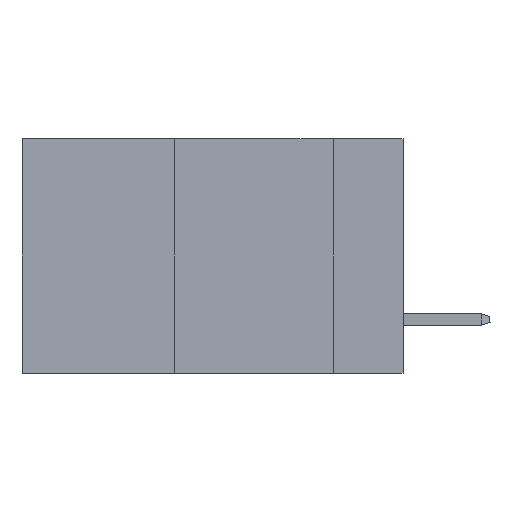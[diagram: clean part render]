
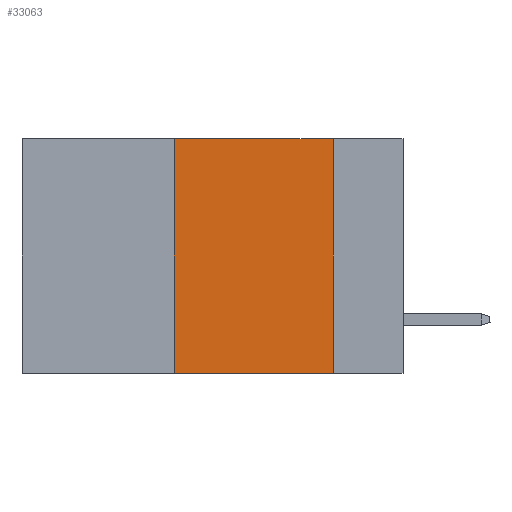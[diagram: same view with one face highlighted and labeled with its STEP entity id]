
A CAD part, left-side view. The second image highlights one B-rep face of the part: STEP entity #33063.
In plain terms, the highlighted planar face has unit normal (-1, 0, 0).
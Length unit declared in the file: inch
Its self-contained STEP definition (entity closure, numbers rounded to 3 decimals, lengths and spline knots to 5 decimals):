
#2587 = AXIS2_PLACEMENT_3D ( 'NONE', #7701, #29586, #21492 ) ;
#3029 = CARTESIAN_POINT ( 'NONE',  ( 0., 0.36, -0.37 ) ) ;
#4555 = ORIENTED_EDGE ( 'NONE', *, *, #9800, .F. ) ;
#4723 = VECTOR ( 'NONE', #30569, 39.37008 ) ;
#5368 = DIRECTION ( 'NONE',  ( 0., -1., 0. ) ) ;
#7594 = VERTEX_POINT ( 'NONE', #3029 ) ;
#7701 = CARTESIAN_POINT ( 'NONE',  ( 0., 0.6, 0. ) ) ;
#7970 = DIRECTION ( 'NONE',  ( 0., 0., 1. ) ) ;
#8715 = CARTESIAN_POINT ( 'NONE',  ( 0., 0.36, 0. ) ) ;
#9434 = VECTOR ( 'NONE', #33396, 39.37008 ) ;
#9800 = EDGE_CURVE ( 'NONE', #7594, #21122, #24262, .T. ) ;
#10902 = CARTESIAN_POINT ( 'NONE',  ( 0., 0.11, -0.37 ) ) ;
#12547 = EDGE_CURVE ( 'NONE', #25622, #34567, #19617, .T. ) ;
#13004 = CARTESIAN_POINT ( 'NONE',  ( 0., 0.36, 0. ) ) ;
#13095 = FACE_OUTER_BOUND ( 'NONE', #35415, .T. ) ;
#13695 = ORIENTED_EDGE ( 'NONE', *, *, #12547, .F. ) ;
#14243 = CARTESIAN_POINT ( 'NONE',  ( 0., 0.11, 0. ) ) ;
#15409 = EDGE_CURVE ( 'NONE', #21122, #25622, #27994, .T. ) ;
#17820 = VECTOR ( 'NONE', #7970, 39.37008 ) ;
#19617 = LINE ( 'NONE', #14243, #4723 ) ;
#19908 = CARTESIAN_POINT ( 'NONE',  ( 0., 0.6, 0. ) ) ;
#20350 = ORIENTED_EDGE ( 'NONE', *, *, #15409, .F. ) ;
#21122 = VERTEX_POINT ( 'NONE', #8715 ) ;
#21323 = PLANE ( 'NONE',  #2587 ) ;
#21492 = DIRECTION ( 'NONE',  ( 0., 0., -1. ) ) ;
#24262 = LINE ( 'NONE', #13004, #17820 ) ;
#25587 = ORIENTED_EDGE ( 'NONE', *, *, #33026, .T. ) ;
#25622 = VERTEX_POINT ( 'NONE', #27530 ) ;
#27530 = CARTESIAN_POINT ( 'NONE',  ( 0., 0.11, 0. ) ) ;
#27994 = LINE ( 'NONE', #19908, #9434 ) ;
#29586 = DIRECTION ( 'NONE',  ( 1., 0., 0. ) ) ;
#29944 = CARTESIAN_POINT ( 'NONE',  ( 0., 0.6, -0.37 ) ) ;
#30569 = DIRECTION ( 'NONE',  ( 0., 0., -1. ) ) ;
#31232 = VECTOR ( 'NONE', #5368, 39.37008 ) ;
#33026 = EDGE_CURVE ( 'NONE', #7594, #34567, #35164, .T. ) ;
#33063 = ADVANCED_FACE ( 'NONE', ( #13095 ), #21323, .F. ) ;
#33396 = DIRECTION ( 'NONE',  ( 0., -1., 0. ) ) ;
#34567 = VERTEX_POINT ( 'NONE', #10902 ) ;
#35164 = LINE ( 'NONE', #29944, #31232 ) ;
#35415 = EDGE_LOOP ( 'NONE', ( #13695, #20350, #4555, #25587 ) ) ;
